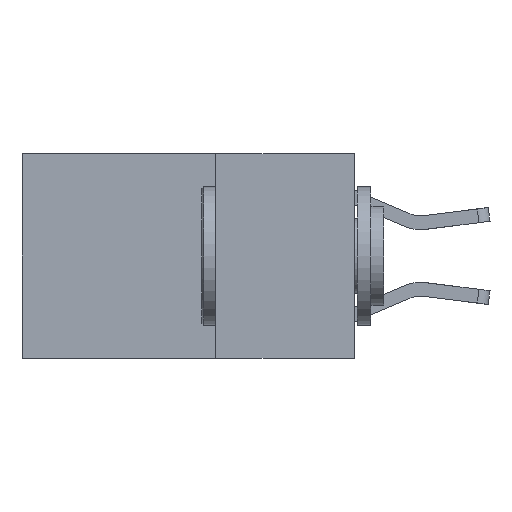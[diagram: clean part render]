
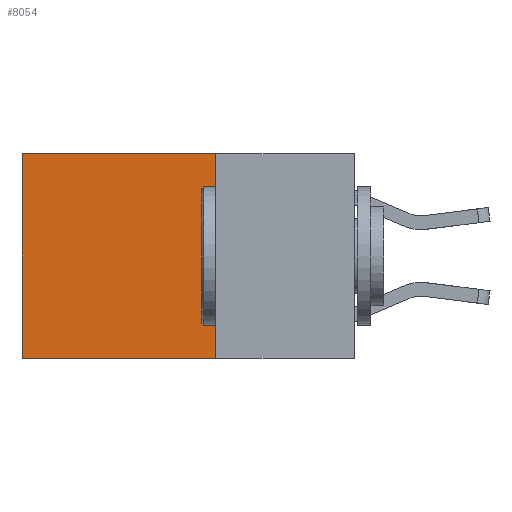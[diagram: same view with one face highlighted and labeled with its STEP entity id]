
A CAD part, left-side view. The second image highlights one B-rep face of the part: STEP entity #8054.
In plain terms, the highlighted planar face has unit normal (-1, 0, 0).
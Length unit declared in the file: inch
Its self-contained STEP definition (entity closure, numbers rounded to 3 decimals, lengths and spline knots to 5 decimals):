
#302 = DIRECTION ( 'NONE',  ( 0., 1., 0. ) ) ;
#484 = ORIENTED_EDGE ( 'NONE', *, *, #3242, .F. ) ;
#496 = DIRECTION ( 'NONE',  ( 0., 0., -1. ) ) ;
#525 = CARTESIAN_POINT ( 'NONE',  ( 0.2625, 0.25, 0. ) ) ;
#575 = CARTESIAN_POINT ( 'NONE',  ( 0.2625, 0.25, -0.37 ) ) ;
#761 = VERTEX_POINT ( 'NONE', #10370 ) ;
#1142 = VERTEX_POINT ( 'NONE', #5844 ) ;
#1491 = DIRECTION ( 'NONE',  ( 0., 0., -1. ) ) ;
#3223 = CARTESIAN_POINT ( 'NONE',  ( 0.2625, 0.6, 0. ) ) ;
#3242 = EDGE_CURVE ( 'NONE', #1142, #761, #10385, .T. ) ;
#4056 = ORIENTED_EDGE ( 'NONE', *, *, #7185, .T. ) ;
#4309 = DIRECTION ( 'NONE',  ( 0., 0., -1. ) ) ;
#5114 = ORIENTED_EDGE ( 'NONE', *, *, #7139, .F. ) ;
#5206 = LINE ( 'NONE', #6874, #5903 ) ;
#5304 = CARTESIAN_POINT ( 'NONE',  ( 0.2625, 0.25, 0. ) ) ;
#5709 = VECTOR ( 'NONE', #8647, 39.37008 ) ;
#5844 = CARTESIAN_POINT ( 'NONE',  ( 0.2625, 0.25, -0.37 ) ) ;
#5903 = VECTOR ( 'NONE', #4309, 39.37008 ) ;
#5908 = ORIENTED_EDGE ( 'NONE', *, *, #8652, .T. ) ;
#6078 = AXIS2_PLACEMENT_3D ( 'NONE', #9590, #11240, #496 ) ;
#6761 = VECTOR ( 'NONE', #302, 39.37008 ) ;
#6874 = CARTESIAN_POINT ( 'NONE',  ( 0.2625, 0.6, 0. ) ) ;
#7099 = LINE ( 'NONE', #525, #7704 ) ;
#7139 = EDGE_CURVE ( 'NONE', #8791, #1142, #7099, .T. ) ;
#7185 = EDGE_CURVE ( 'NONE', #8791, #8298, #9805, .T. ) ;
#7704 = VECTOR ( 'NONE', #1491, 39.37008 ) ;
#8054 = ADVANCED_FACE ( 'NONE', ( #8817 ), #8638, .F. ) ;
#8298 = VERTEX_POINT ( 'NONE', #3223 ) ;
#8638 = PLANE ( 'NONE',  #6078 ) ;
#8647 = DIRECTION ( 'NONE',  ( 0., 1., 0. ) ) ;
#8652 = EDGE_CURVE ( 'NONE', #8298, #761, #5206, .T. ) ;
#8791 = VERTEX_POINT ( 'NONE', #10063 ) ;
#8817 = FACE_OUTER_BOUND ( 'NONE', #11714, .T. ) ;
#9590 = CARTESIAN_POINT ( 'NONE',  ( 0.2625, 0.25, 0. ) ) ;
#9805 = LINE ( 'NONE', #5304, #6761 ) ;
#10063 = CARTESIAN_POINT ( 'NONE',  ( 0.2625, 0.25, 0. ) ) ;
#10370 = CARTESIAN_POINT ( 'NONE',  ( 0.2625, 0.6, -0.37 ) ) ;
#10385 = LINE ( 'NONE', #575, #5709 ) ;
#11240 = DIRECTION ( 'NONE',  ( 1., 0., 0. ) ) ;
#11714 = EDGE_LOOP ( 'NONE', ( #5908, #484, #5114, #4056 ) ) ;
